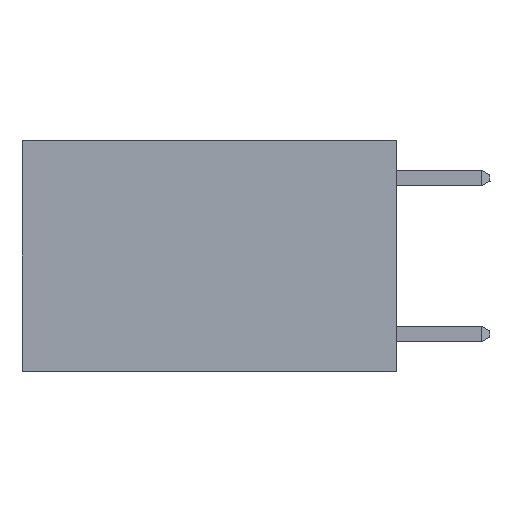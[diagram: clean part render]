
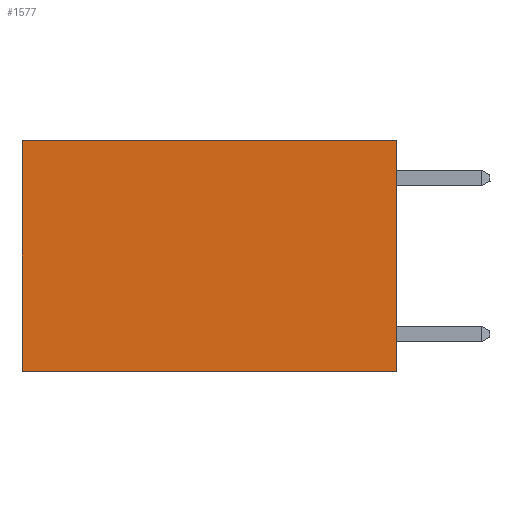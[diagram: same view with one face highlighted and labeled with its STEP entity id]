
A CAD part, left-side view. The second image highlights one B-rep face of the part: STEP entity #1577.
In plain terms, the highlighted planar face has unit normal (-1, 0, 0).
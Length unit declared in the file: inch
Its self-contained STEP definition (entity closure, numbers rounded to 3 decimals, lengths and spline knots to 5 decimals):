
#1101 = VERTEX_POINT ( 'NONE', #13505 ) ;
#1513 = EDGE_CURVE ( 'NONE', #6889, #7647, #15800, .T. ) ;
#1545 = VECTOR ( 'NONE', #5095, 39.37008 ) ;
#1577 = ADVANCED_FACE ( 'NONE', ( #21053 ), #12857, .F. ) ;
#1946 = LINE ( 'NONE', #8136, #21156 ) ;
#2018 = LINE ( 'NONE', #21789, #14549 ) ;
#3283 = ORIENTED_EDGE ( 'NONE', *, *, #6522, .T. ) ;
#4248 = VERTEX_POINT ( 'NONE', #21491 ) ;
#4675 = EDGE_CURVE ( 'NONE', #1101, #6889, #2018, .T. ) ;
#4828 = VECTOR ( 'NONE', #22841, 39.37008 ) ;
#5095 = DIRECTION ( 'NONE',  ( 0., 1., 0. ) ) ;
#5098 = DIRECTION ( 'NONE',  ( 0., 0., -1. ) ) ;
#6522 = EDGE_CURVE ( 'NONE', #4248, #7647, #6601, .T. ) ;
#6601 = LINE ( 'NONE', #9654, #4828 ) ;
#6889 = VERTEX_POINT ( 'NONE', #9544 ) ;
#7647 = VERTEX_POINT ( 'NONE', #16420 ) ;
#8136 = CARTESIAN_POINT ( 'NONE',  ( 0.2625, 0., 0. ) ) ;
#9371 = DIRECTION ( 'NONE',  ( 0., 0., -1. ) ) ;
#9544 = CARTESIAN_POINT ( 'NONE',  ( 0.2625, 0., -0.37 ) ) ;
#9654 = CARTESIAN_POINT ( 'NONE',  ( 0.2625, 0.6, 0. ) ) ;
#9862 = DIRECTION ( 'NONE',  ( 0., 1., 0. ) ) ;
#10715 = CARTESIAN_POINT ( 'NONE',  ( 0.2625, 0., -0.37 ) ) ;
#12857 = PLANE ( 'NONE',  #22458 ) ;
#13183 = ORIENTED_EDGE ( 'NONE', *, *, #20518, .T. ) ;
#13505 = CARTESIAN_POINT ( 'NONE',  ( 0.2625, 0., 0. ) ) ;
#14114 = ORIENTED_EDGE ( 'NONE', *, *, #4675, .F. ) ;
#14549 = VECTOR ( 'NONE', #5098, 39.37008 ) ;
#15800 = LINE ( 'NONE', #10715, #1545 ) ;
#16420 = CARTESIAN_POINT ( 'NONE',  ( 0.2625, 0.6, -0.37 ) ) ;
#18457 = DIRECTION ( 'NONE',  ( 1., 0., 0. ) ) ;
#20334 = EDGE_LOOP ( 'NONE', ( #3283, #22256, #14114, #13183 ) ) ;
#20518 = EDGE_CURVE ( 'NONE', #1101, #4248, #1946, .T. ) ;
#20630 = CARTESIAN_POINT ( 'NONE',  ( 0.2625, 0., 0. ) ) ;
#21053 = FACE_OUTER_BOUND ( 'NONE', #20334, .T. ) ;
#21156 = VECTOR ( 'NONE', #9862, 39.37008 ) ;
#21491 = CARTESIAN_POINT ( 'NONE',  ( 0.2625, 0.6, 0. ) ) ;
#21789 = CARTESIAN_POINT ( 'NONE',  ( 0.2625, 0., 0. ) ) ;
#22256 = ORIENTED_EDGE ( 'NONE', *, *, #1513, .F. ) ;
#22458 = AXIS2_PLACEMENT_3D ( 'NONE', #20630, #18457, #9371 ) ;
#22841 = DIRECTION ( 'NONE',  ( 0., 0., -1. ) ) ;
